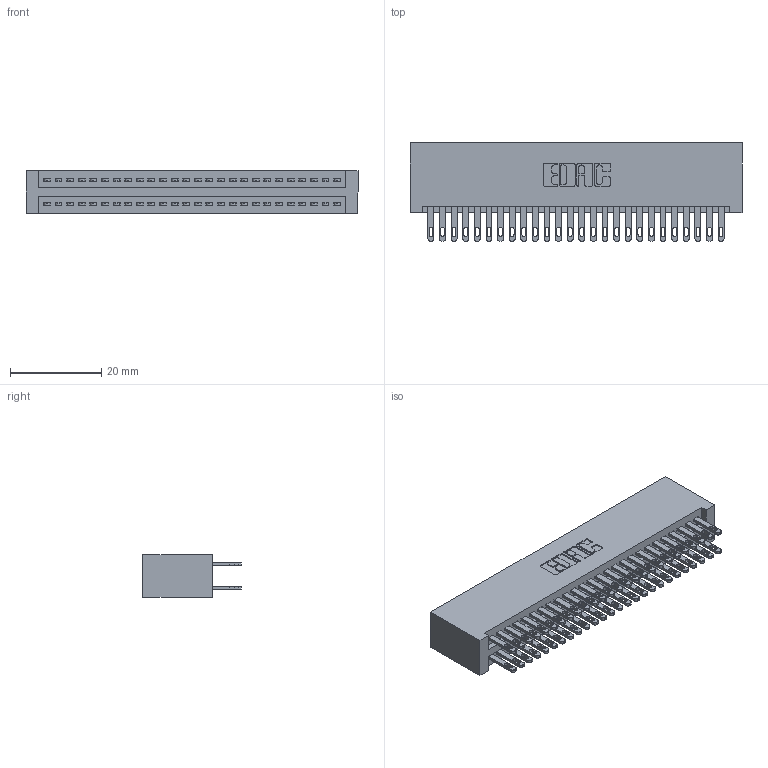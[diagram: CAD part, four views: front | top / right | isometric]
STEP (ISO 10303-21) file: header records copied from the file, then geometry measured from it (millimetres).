
FILE_DESCRIPTION (( 'STEP AP203' ), '1' );
FILE_NAME ('895-052-500-201.STEP', '2020-09-27T10:55:10', ( '' ), ( '' ), 'SwSTEP 2.0', 'SolidWorks 2020', '' );
FILE_SCHEMA (( 'CONFIG_CONTROL_DESIGN' ));
Length unit declared in the file: inch
Products named in the file (3): 845 Part_No Mounting Lugs; 895-052-500-201; 345-292-001_345-293-100
Assembly tree (53 placements, depth 2):
  895-052-500-201
    845 Part_No Mounting Lugs
    345-292-001_345-293-100  x52
Bounding box: 72.64 x 21.51 x 9.4 mm (x, y, z)
Volume: 7683 mm3; surface area: 11880.5 mm2
Topology: 53 solids, 53 shells, 2510 faces, 7649 edges, 5098 vertices
Faces by surface type: plane 1480, cylinder 1030
Entity records: 22207 total; most frequent: CARTESIAN_POINT 3736, ORIENTED_EDGE 3670, DIRECTION 3311, EDGE_CURVE 1835, LINE 1603, VECTOR 1603, VERTEX_POINT 1222, AXIS2_PLACEMENT_3D 854
